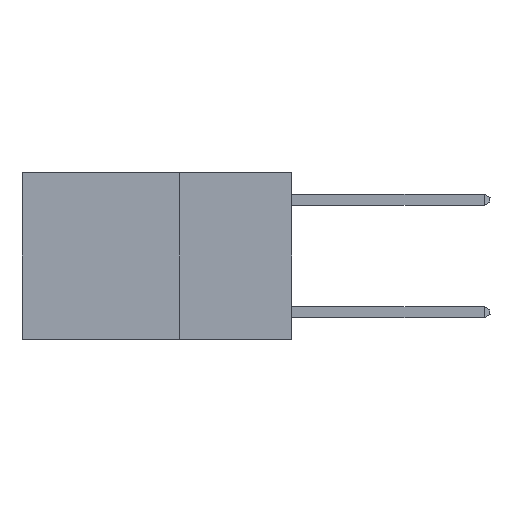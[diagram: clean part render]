
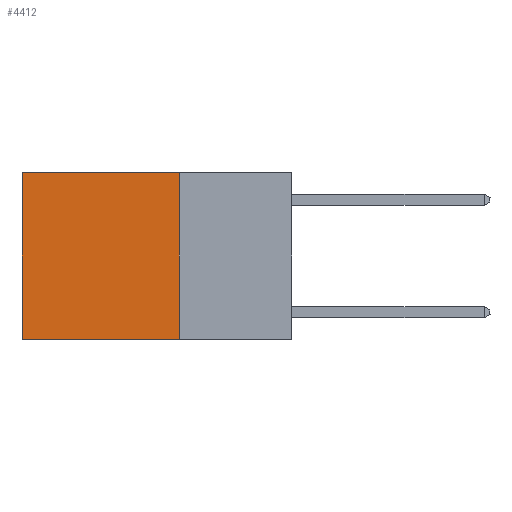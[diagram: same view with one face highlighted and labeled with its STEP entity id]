
A CAD part, left-side view. The second image highlights one B-rep face of the part: STEP entity #4412.
In plain terms, the highlighted planar face has unit normal (-1, 0, 0).
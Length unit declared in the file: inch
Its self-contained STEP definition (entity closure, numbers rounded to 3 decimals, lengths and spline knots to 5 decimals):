
#889 = LINE ( 'NONE', #6412, #1552 ) ;
#1552 = VECTOR ( 'NONE', #15069, 39.37008 ) ;
#3588 = VECTOR ( 'NONE', #15936, 39.37008 ) ;
#3727 = FACE_OUTER_BOUND ( 'NONE', #17958, .T. ) ;
#3952 = EDGE_CURVE ( 'NONE', #12740, #14348, #889, .T. ) ;
#3993 = DIRECTION ( 'NONE',  ( 0., 0., -1. ) ) ;
#4412 = ADVANCED_FACE ( 'NONE', ( #3727 ), #12341, .F. ) ;
#4547 = LINE ( 'NONE', #11425, #3588 ) ;
#5019 = CARTESIAN_POINT ( 'NONE',  ( 0.2625, 0.25, -0.37 ) ) ;
#6412 = CARTESIAN_POINT ( 'NONE',  ( 0.2625, 0.25, 0. ) ) ;
#6881 = VERTEX_POINT ( 'NONE', #7329 ) ;
#7084 = ORIENTED_EDGE ( 'NONE', *, *, #11834, .F. ) ;
#7329 = CARTESIAN_POINT ( 'NONE',  ( 0.2625, 0.6, 0. ) ) ;
#8343 = DIRECTION ( 'NONE',  ( 0., 1., 0. ) ) ;
#9207 = ORIENTED_EDGE ( 'NONE', *, *, #3952, .F. ) ;
#9934 = CARTESIAN_POINT ( 'NONE',  ( 0.2625, 0.6, -0.37 ) ) ;
#10069 = LINE ( 'NONE', #14583, #12315 ) ;
#10310 = VERTEX_POINT ( 'NONE', #9934 ) ;
#10617 = DIRECTION ( 'NONE',  ( 0., 1., 0. ) ) ;
#10706 = EDGE_CURVE ( 'NONE', #12740, #6881, #10069, .T. ) ;
#10757 = CARTESIAN_POINT ( 'NONE',  ( 0.2625, 0.25, 0. ) ) ;
#11071 = CARTESIAN_POINT ( 'NONE',  ( 0.2625, 0.25, -0.37 ) ) ;
#11425 = CARTESIAN_POINT ( 'NONE',  ( 0.2625, 0.6, 0. ) ) ;
#11834 = EDGE_CURVE ( 'NONE', #14348, #10310, #11983, .T. ) ;
#11983 = LINE ( 'NONE', #5019, #16742 ) ;
#12315 = VECTOR ( 'NONE', #8343, 39.37008 ) ;
#12341 = PLANE ( 'NONE',  #12730 ) ;
#12730 = AXIS2_PLACEMENT_3D ( 'NONE', #15023, #13440, #3993 ) ;
#12740 = VERTEX_POINT ( 'NONE', #10757 ) ;
#13440 = DIRECTION ( 'NONE',  ( 1., 0., 0. ) ) ;
#13470 = EDGE_CURVE ( 'NONE', #6881, #10310, #4547, .T. ) ;
#14348 = VERTEX_POINT ( 'NONE', #11071 ) ;
#14583 = CARTESIAN_POINT ( 'NONE',  ( 0.2625, 0.25, 0. ) ) ;
#15023 = CARTESIAN_POINT ( 'NONE',  ( 0.2625, 0.25, 0. ) ) ;
#15069 = DIRECTION ( 'NONE',  ( 0., 0., -1. ) ) ;
#15122 = ORIENTED_EDGE ( 'NONE', *, *, #13470, .T. ) ;
#15936 = DIRECTION ( 'NONE',  ( 0., 0., -1. ) ) ;
#16742 = VECTOR ( 'NONE', #10617, 39.37008 ) ;
#17176 = ORIENTED_EDGE ( 'NONE', *, *, #10706, .T. ) ;
#17958 = EDGE_LOOP ( 'NONE', ( #15122, #7084, #9207, #17176 ) ) ;
